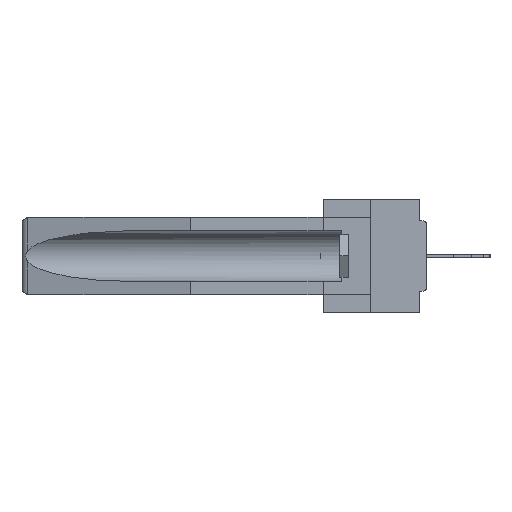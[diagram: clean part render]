
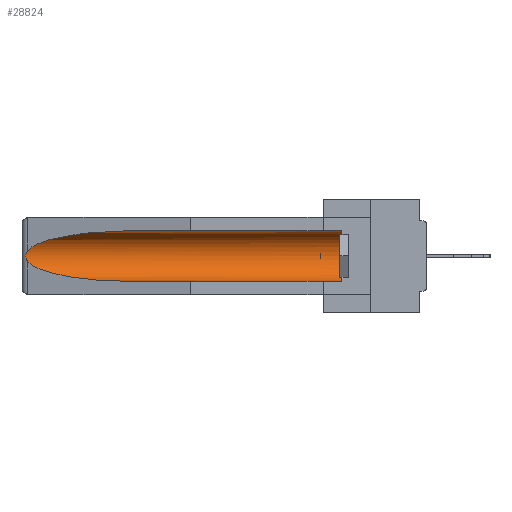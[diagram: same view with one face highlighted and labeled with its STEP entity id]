
A CAD part, left-side view. The second image highlights one B-rep face of the part: STEP entity #28824.
In plain terms, the highlighted cylindrical face has radius 2.857 mm (diameter 5.715 mm), a partial arc.
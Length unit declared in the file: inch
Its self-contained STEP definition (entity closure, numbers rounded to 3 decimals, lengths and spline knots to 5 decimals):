
#535 = CARTESIAN_POINT ( 'NONE',  ( 0.26597, 1.52961, -0.15275 ) ) ;
#946 = CARTESIAN_POINT ( 'NONE',  ( 0.155, 1.07973, -0.059 ) ) ;
#1189 = DIRECTION ( 'NONE',  ( 0., 1., 0. ) ) ;
#1321 = ORIENTED_EDGE ( 'NONE', *, *, #17551, .T. ) ;
#1359 = CARTESIAN_POINT ( 'NONE',  ( 0.21114, 1.30732, -0.059 ) ) ;
#1729 = B_SPLINE_CURVE_WITH_KNOTS ( 'NONE', 3,
 ( #22924, #535, #33271, #39113, #19281, #9593, #22712, #36507, #23140, #42549 ),
 .UNSPECIFIED., .F., .F.,
 ( 4, 2, 2, 2, 4 ),
 ( 0., 0.00029, 0.00058, 0.00087, 0.00117 ),
 .UNSPECIFIED. ) ;
#3105 = VERTEX_POINT ( 'NONE', #17075 ) ;
#4075 = CARTESIAN_POINT ( 'NONE',  ( 0.155, -0.30754, -0.1715 ) ) ;
#4571 = VERTEX_POINT ( 'NONE', #4783 ) ;
#4783 = CARTESIAN_POINT ( 'NONE',  ( 0.155, 0.126, -0.059 ) ) ;
#5727 = DIRECTION ( 'NONE',  ( 0., -1., 0. ) ) ;
#6879 = VERTEX_POINT ( 'NONE', #7246 ) ;
#7232 = LINE ( 'NONE', #27029, #36661 ) ;
#7246 = CARTESIAN_POINT ( 'NONE',  ( 0.155, 0.126, -0.284 ) ) ;
#8260 = EDGE_CURVE ( 'NONE', #3105, #31071, #31546, .T. ) ;
#8320 = EDGE_CURVE ( 'NONE', #6879, #4571, #38256, .T. ) ;
#9593 = CARTESIAN_POINT ( 'NONE',  ( 0.2675, 1.53308, -0.17534 ) ) ;
#10754 = FACE_OUTER_BOUND ( 'NONE', #26999, .T. ) ;
#10966 = DIRECTION ( 'NONE',  ( 0., 1., 0. ) ) ;
#11272 = CARTESIAN_POINT ( 'NONE',  ( 0.25451, 1.48313, -0.09465 ) ) ;
#13230 = ORIENTED_EDGE ( 'NONE', *, *, #15949, .F. ) ;
#15625 = CARTESIAN_POINT ( 'NONE',  ( 0.155, -0.30754, -0.284 ) ) ;
#15949 = EDGE_CURVE ( 'NONE', #6879, #31071, #35432, .T. ) ;
#17075 = CARTESIAN_POINT ( 'NONE',  ( 0.26537, 1.52718, -0.19328 ) ) ;
#17325 = CARTESIAN_POINT ( 'NONE',  ( 0.155, 1.07973, -0.059 ) ) ;
#17551 = EDGE_CURVE ( 'NONE', #37215, #28245, #30164, .T. ) ;
#19281 = CARTESIAN_POINT ( 'NONE',  ( 0.2675, 1.53308, -0.16763 ) ) ;
#19566 = ORIENTED_EDGE ( 'NONE', *, *, #39776, .T. ) ;
#20656 = CYLINDRICAL_SURFACE ( 'NONE', #42346, 0.1125 ) ;
#21020 = CARTESIAN_POINT ( 'NONE',  ( 0.21114, 1.30732, -0.284 ) ) ;
#22062 = DIRECTION ( 'NONE',  ( 0., 1., 0. ) ) ;
#22712 = CARTESIAN_POINT ( 'NONE',  ( 0.2673, 1.53269, -0.17917 ) ) ;
#22924 = CARTESIAN_POINT ( 'NONE',  ( 0.26537, 1.52718, -0.14972 ) ) ;
#23140 = CARTESIAN_POINT ( 'NONE',  ( 0.26597, 1.5296, -0.19026 ) ) ;
#23651 = DIRECTION ( 'NONE',  ( 0., 0., 1. ) ) ;
#24239 = CARTESIAN_POINT ( 'NONE',  ( 0.155, 1.07973, -0.284 ) ) ;
#24394 = CARTESIAN_POINT ( 'NONE',  ( 0.26537, 1.52718, -0.14972 ) ) ;
#24663 = DIRECTION ( 'NONE',  ( 0., 0., 1. ) ) ;
#25251 = VECTOR ( 'NONE', #22062, 39.37008 ) ;
#26999 = EDGE_LOOP ( 'NONE', ( #1321, #30435, #29729, #13230, #37223, #19566 ) ) ;
#27029 = CARTESIAN_POINT ( 'NONE',  ( 0.155, -0.30754, -0.059 ) ) ;
#28245 = VERTEX_POINT ( 'NONE', #39055 ) ;
#28824 = ADVANCED_FACE ( 'NONE', ( #10754 ), #20656, .F. ) ;
#29729 = ORIENTED_EDGE ( 'NONE', *, *, #8260, .T. ) ;
#30164 =( BOUNDED_CURVE ( )  B_SPLINE_CURVE ( 3, ( #946, #1359, #11272, #24394 ),
 .UNSPECIFIED., .F., .F. ) 
 B_SPLINE_CURVE_WITH_KNOTS ( ( 4, 4 ),
 ( 4.71239, 6.08839 ),
 .UNSPECIFIED. ) 
 CURVE ( )  GEOMETRIC_REPRESENTATION_ITEM ( )  RATIONAL_B_SPLINE_CURVE ( ( 1., 0.848, 0.848, 1. ) ) 
 REPRESENTATION_ITEM ( '' )  );
#30435 = ORIENTED_EDGE ( 'NONE', *, *, #37073, .T. ) ;
#31071 = VERTEX_POINT ( 'NONE', #36652 ) ;
#31140 = CARTESIAN_POINT ( 'NONE',  ( 0.26537, 1.52718, -0.19328 ) ) ;
#31546 =( BOUNDED_CURVE ( )  B_SPLINE_CURVE ( 3, ( #31140, #40624, #21020, #24239 ),
 .UNSPECIFIED., .F., .F. ) 
 B_SPLINE_CURVE_WITH_KNOTS ( ( 4, 4 ),
 ( 0.1948, 1.5708 ),
 .UNSPECIFIED. ) 
 CURVE ( )  GEOMETRIC_REPRESENTATION_ITEM ( )  RATIONAL_B_SPLINE_CURVE ( ( 1., 0.848, 0.848, 1. ) ) 
 REPRESENTATION_ITEM ( '' )  );
#33271 = CARTESIAN_POINT ( 'NONE',  ( 0.26654, 1.53092, -0.15636 ) ) ;
#34809 = CARTESIAN_POINT ( 'NONE',  ( 0.155, 0.126, -0.1715 ) ) ;
#35432 = LINE ( 'NONE', #15625, #25251 ) ;
#36227 = AXIS2_PLACEMENT_3D ( 'NONE', #34809, #5727, #24663 ) ;
#36507 = CARTESIAN_POINT ( 'NONE',  ( 0.26655, 1.53094, -0.18657 ) ) ;
#36652 = CARTESIAN_POINT ( 'NONE',  ( 0.155, 1.07973, -0.284 ) ) ;
#36661 = VECTOR ( 'NONE', #1189, 39.37008 ) ;
#37073 = EDGE_CURVE ( 'NONE', #28245, #3105, #1729, .T. ) ;
#37215 = VERTEX_POINT ( 'NONE', #17325 ) ;
#37223 = ORIENTED_EDGE ( 'NONE', *, *, #8320, .T. ) ;
#38256 = CIRCLE ( 'NONE', #36227, 0.1125 ) ;
#39055 = CARTESIAN_POINT ( 'NONE',  ( 0.26537, 1.52718, -0.14972 ) ) ;
#39113 = CARTESIAN_POINT ( 'NONE',  ( 0.2673, 1.5327, -0.16383 ) ) ;
#39776 = EDGE_CURVE ( 'NONE', #4571, #37215, #7232, .T. ) ;
#40624 = CARTESIAN_POINT ( 'NONE',  ( 0.25451, 1.48313, -0.24835 ) ) ;
#42346 = AXIS2_PLACEMENT_3D ( 'NONE', #4075, #10966, #23651 ) ;
#42549 = CARTESIAN_POINT ( 'NONE',  ( 0.26537, 1.52718, -0.19328 ) ) ;
